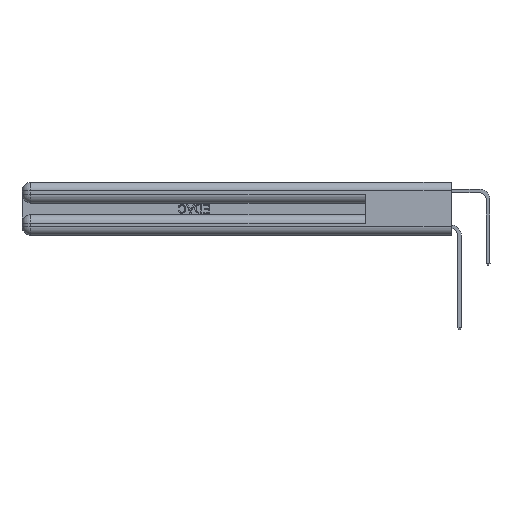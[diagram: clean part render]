
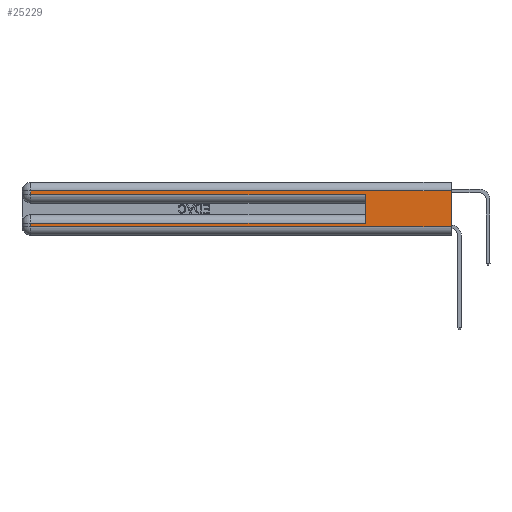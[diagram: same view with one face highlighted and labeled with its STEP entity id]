
A CAD part, left-side view. The second image highlights one B-rep face of the part: STEP entity #25229.
In plain terms, the highlighted planar face has unit normal (-1, 0, 0).
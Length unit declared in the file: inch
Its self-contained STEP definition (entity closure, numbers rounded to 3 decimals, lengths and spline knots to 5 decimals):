
#2 = DIRECTION ( 'NONE',  ( 0., 1., 0. ) ) ;
#699 = CARTESIAN_POINT ( 'NONE',  ( 0., 0.6, 0.145 ) ) ;
#766 = CARTESIAN_POINT ( 'NONE',  ( 0., 2.94, 0.31 ) ) ;
#1055 = EDGE_CURVE ( 'NONE', #13533, #26432, #10620, .T. ) ;
#2235 = VERTEX_POINT ( 'NONE', #25059 ) ;
#2666 = CARTESIAN_POINT ( 'NONE',  ( 0., 0., 0.06 ) ) ;
#2763 = LINE ( 'NONE', #24033, #18992 ) ;
#3127 = VERTEX_POINT ( 'NONE', #766 ) ;
#3414 = ORIENTED_EDGE ( 'NONE', *, *, #15505, .T. ) ;
#3836 = LINE ( 'NONE', #6158, #22418 ) ;
#4299 = PLANE ( 'NONE',  #27450 ) ;
#4394 = DIRECTION ( 'NONE',  ( 0., -1., 0. ) ) ;
#4506 = EDGE_CURVE ( 'NONE', #14722, #21249, #22043, .T. ) ;
#4840 = LINE ( 'NONE', #5290, #10292 ) ;
#5290 = CARTESIAN_POINT ( 'NONE',  ( 0., 2.94, 0.37 ) ) ;
#6158 = CARTESIAN_POINT ( 'NONE',  ( 0., 0., 0.285 ) ) ;
#7411 = CARTESIAN_POINT ( 'NONE',  ( 0., 0., 0.31 ) ) ;
#8137 = LINE ( 'NONE', #699, #29017 ) ;
#8498 = DIRECTION ( 'NONE',  ( 0., 0., -1. ) ) ;
#8576 = ORIENTED_EDGE ( 'NONE', *, *, #17719, .F. ) ;
#8766 = CARTESIAN_POINT ( 'NONE',  ( 0., 0., 0.37 ) ) ;
#10292 = VECTOR ( 'NONE', #14293, 39.37008 ) ;
#10555 = CARTESIAN_POINT ( 'NONE',  ( 0., 0., 0.06 ) ) ;
#10620 = LINE ( 'NONE', #8766, #22897 ) ;
#10705 = VECTOR ( 'NONE', #4394, 39.37008 ) ;
#10975 = CARTESIAN_POINT ( 'NONE',  ( 0., 0., 0.37 ) ) ;
#11295 = ORIENTED_EDGE ( 'NONE', *, *, #23071, .T. ) ;
#12274 = VECTOR ( 'NONE', #17692, 39.37008 ) ;
#13212 = CARTESIAN_POINT ( 'NONE',  ( 0., 0.6, 0.285 ) ) ;
#13533 = VERTEX_POINT ( 'NONE', #26046 ) ;
#14119 = EDGE_CURVE ( 'NONE', #2235, #27742, #3836, .T. ) ;
#14293 = DIRECTION ( 'NONE',  ( 0., 0., -1. ) ) ;
#14722 = VERTEX_POINT ( 'NONE', #26765 ) ;
#15497 = EDGE_CURVE ( 'NONE', #13533, #3127, #23438, .T. ) ;
#15505 = EDGE_CURVE ( 'NONE', #3127, #2235, #2763, .T. ) ;
#15904 = VERTEX_POINT ( 'NONE', #21641 ) ;
#16113 = FACE_OUTER_BOUND ( 'NONE', #20692, .T. ) ;
#16185 = ORIENTED_EDGE ( 'NONE', *, *, #4506, .T. ) ;
#17529 = CARTESIAN_POINT ( 'NONE',  ( 0., 0., 0.085 ) ) ;
#17692 = DIRECTION ( 'NONE',  ( 0., 1., 0. ) ) ;
#17719 = EDGE_CURVE ( 'NONE', #14722, #27742, #8137, .T. ) ;
#18006 = ORIENTED_EDGE ( 'NONE', *, *, #15497, .T. ) ;
#18992 = VECTOR ( 'NONE', #21716, 39.37008 ) ;
#19741 = ORIENTED_EDGE ( 'NONE', *, *, #14119, .T. ) ;
#20110 = DIRECTION ( 'NONE',  ( 0., 0., 1. ) ) ;
#20692 = EDGE_LOOP ( 'NONE', ( #23467, #18006, #3414, #19741, #8576, #16185, #11295, #29629 ) ) ;
#21249 = VERTEX_POINT ( 'NONE', #29903 ) ;
#21641 = CARTESIAN_POINT ( 'NONE',  ( 0., 2.94, 0.06 ) ) ;
#21716 = DIRECTION ( 'NONE',  ( 0., 0., -1. ) ) ;
#22043 = LINE ( 'NONE', #17529, #12274 ) ;
#22418 = VECTOR ( 'NONE', #29480, 39.37008 ) ;
#22897 = VECTOR ( 'NONE', #23230, 39.37008 ) ;
#23071 = EDGE_CURVE ( 'NONE', #21249, #15904, #4840, .T. ) ;
#23230 = DIRECTION ( 'NONE',  ( 0., 0., -1. ) ) ;
#23270 = DIRECTION ( 'NONE',  ( 1., 0., 0. ) ) ;
#23438 = LINE ( 'NONE', #7411, #28925 ) ;
#23467 = ORIENTED_EDGE ( 'NONE', *, *, #1055, .F. ) ;
#24033 = CARTESIAN_POINT ( 'NONE',  ( 0., 2.94, 0.37 ) ) ;
#25059 = CARTESIAN_POINT ( 'NONE',  ( 0., 2.94, 0.285 ) ) ;
#25229 = ADVANCED_FACE ( 'NONE', ( #16113 ), #4299, .F. ) ;
#26046 = CARTESIAN_POINT ( 'NONE',  ( 0., 0., 0.31 ) ) ;
#26432 = VERTEX_POINT ( 'NONE', #10555 ) ;
#26765 = CARTESIAN_POINT ( 'NONE',  ( 0., 0.6, 0.085 ) ) ;
#27450 = AXIS2_PLACEMENT_3D ( 'NONE', #10975, #23270, #8498 ) ;
#27742 = VERTEX_POINT ( 'NONE', #13212 ) ;
#28316 = LINE ( 'NONE', #2666, #10705 ) ;
#28925 = VECTOR ( 'NONE', #2, 39.37008 ) ;
#29017 = VECTOR ( 'NONE', #20110, 39.37008 ) ;
#29480 = DIRECTION ( 'NONE',  ( 0., -1., 0. ) ) ;
#29629 = ORIENTED_EDGE ( 'NONE', *, *, #30612, .T. ) ;
#29903 = CARTESIAN_POINT ( 'NONE',  ( 0., 2.94, 0.085 ) ) ;
#30612 = EDGE_CURVE ( 'NONE', #15904, #26432, #28316, .T. ) ;
